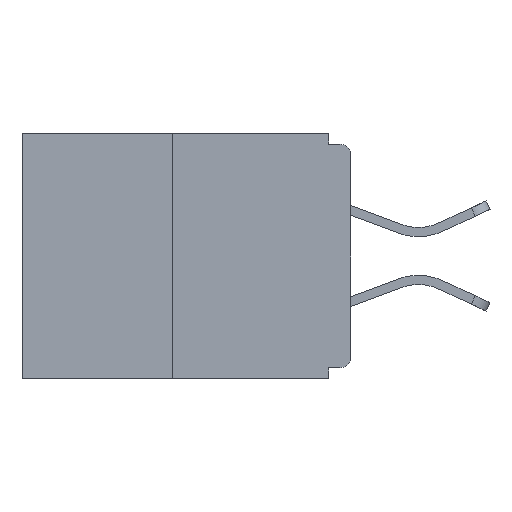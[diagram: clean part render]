
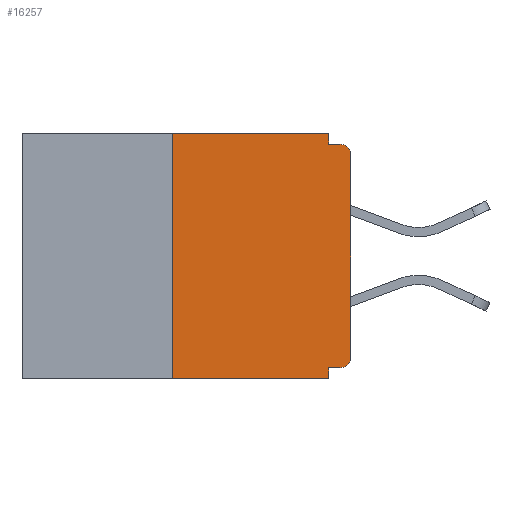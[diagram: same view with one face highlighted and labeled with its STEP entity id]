
A CAD part, left-side view. The second image highlights one B-rep face of the part: STEP entity #16257.
In plain terms, the highlighted planar face has unit normal (-1, 0, 0).
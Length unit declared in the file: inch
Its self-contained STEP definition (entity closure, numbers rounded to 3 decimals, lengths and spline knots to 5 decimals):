
#686 = CARTESIAN_POINT ( 'NONE',  ( 0., 0.015, -0.03 ) ) ;
#1086 = LINE ( 'NONE', #7236, #3591 ) ;
#1293 = LINE ( 'NONE', #18063, #6574 ) ;
#1392 = VERTEX_POINT ( 'NONE', #3799 ) ;
#1518 = VERTEX_POINT ( 'NONE', #22064 ) ;
#2824 = DIRECTION ( 'NONE',  ( 0., -1., 0. ) ) ;
#2896 = CARTESIAN_POINT ( 'NONE',  ( 0., 0.25, 0. ) ) ;
#3111 = EDGE_LOOP ( 'NONE', ( #5064, #6084, #10311, #18192, #11988, #22037, #6986, #12767, #12832, #10343 ) ) ;
#3137 = CARTESIAN_POINT ( 'NONE',  ( 0., 0.46, 0. ) ) ;
#3256 = DIRECTION ( 'NONE',  ( 0., -1., 0. ) ) ;
#3439 = VECTOR ( 'NONE', #3256, 39.37008 ) ;
#3578 = VERTEX_POINT ( 'NONE', #11507 ) ;
#3591 = VECTOR ( 'NONE', #17763, 39.37008 ) ;
#3665 = CIRCLE ( 'NONE', #6596, 0.015 ) ;
#3799 = CARTESIAN_POINT ( 'NONE',  ( 0., 0.015, -0.015 ) ) ;
#3884 = VERTEX_POINT ( 'NONE', #17634 ) ;
#4824 = LINE ( 'NONE', #15716, #3439 ) ;
#5027 = CIRCLE ( 'NONE', #20425, 0.015 ) ;
#5064 = ORIENTED_EDGE ( 'NONE', *, *, #16076, .F. ) ;
#5267 = CARTESIAN_POINT ( 'NONE',  ( 0., 0., -0.015 ) ) ;
#6084 = ORIENTED_EDGE ( 'NONE', *, *, #14226, .F. ) ;
#6134 = VERTEX_POINT ( 'NONE', #9829 ) ;
#6143 = VERTEX_POINT ( 'NONE', #20132 ) ;
#6296 = VERTEX_POINT ( 'NONE', #13304 ) ;
#6304 = LINE ( 'NONE', #5267, #15314 ) ;
#6574 = VECTOR ( 'NONE', #15235, 39.37008 ) ;
#6596 = AXIS2_PLACEMENT_3D ( 'NONE', #21957, #20246, #11429 ) ;
#6986 = ORIENTED_EDGE ( 'NONE', *, *, #22773, .T. ) ;
#7236 = CARTESIAN_POINT ( 'NONE',  ( 0., 0., 0. ) ) ;
#7850 = DIRECTION ( 'NONE',  ( 0., 0., -1. ) ) ;
#8027 = DIRECTION ( 'NONE',  ( -1., 0., 0. ) ) ;
#8207 = DIRECTION ( 'NONE',  ( 0., 0., -1. ) ) ;
#9172 = DIRECTION ( 'NONE',  ( 0., 0., 1. ) ) ;
#9654 = LINE ( 'NONE', #3137, #20111 ) ;
#9720 = EDGE_CURVE ( 'NONE', #6143, #1392, #6304, .T. ) ;
#9829 = CARTESIAN_POINT ( 'NONE',  ( 0., 0.015, -0.328 ) ) ;
#10311 = ORIENTED_EDGE ( 'NONE', *, *, #19846, .T. ) ;
#10343 = ORIENTED_EDGE ( 'NONE', *, *, #17300, .F. ) ;
#11187 = VERTEX_POINT ( 'NONE', #13243 ) ;
#11429 = DIRECTION ( 'NONE',  ( 0., 0., -1. ) ) ;
#11507 = CARTESIAN_POINT ( 'NONE',  ( 0., 0.031, 0. ) ) ;
#11532 = PLANE ( 'NONE',  #16523 ) ;
#11988 = ORIENTED_EDGE ( 'NONE', *, *, #12047, .F. ) ;
#12047 = EDGE_CURVE ( 'NONE', #6134, #3884, #17233, .T. ) ;
#12199 = DIRECTION ( 'NONE',  ( 0., 1., 0. ) ) ;
#12627 = CARTESIAN_POINT ( 'NONE',  ( 0., 0.031, -0.343 ) ) ;
#12767 = ORIENTED_EDGE ( 'NONE', *, *, #21464, .T. ) ;
#12832 = ORIENTED_EDGE ( 'NONE', *, *, #9720, .F. ) ;
#13243 = CARTESIAN_POINT ( 'NONE',  ( 0., 0.25, -0.343 ) ) ;
#13304 = CARTESIAN_POINT ( 'NONE',  ( 0., 0., -0.03 ) ) ;
#13454 = FACE_OUTER_BOUND ( 'NONE', #3111, .T. ) ;
#13843 = VERTEX_POINT ( 'NONE', #12627 ) ;
#14226 = EDGE_CURVE ( 'NONE', #11187, #16064, #19319, .T. ) ;
#15235 = DIRECTION ( 'NONE',  ( 0., 0., -1. ) ) ;
#15314 = VECTOR ( 'NONE', #15618, 39.37008 ) ;
#15618 = DIRECTION ( 'NONE',  ( 0., -1., 0. ) ) ;
#15716 = CARTESIAN_POINT ( 'NONE',  ( 0., 0.46, -0.343 ) ) ;
#16064 = VERTEX_POINT ( 'NONE', #2896 ) ;
#16076 = EDGE_CURVE ( 'NONE', #16064, #3578, #9654, .T. ) ;
#16257 = ADVANCED_FACE ( 'NONE', ( #13454 ), #11532, .F. ) ;
#16523 = AXIS2_PLACEMENT_3D ( 'NONE', #20359, #16613, #7850 ) ;
#16613 = DIRECTION ( 'NONE',  ( 1., 0., 0. ) ) ;
#16784 = DIRECTION ( 'NONE',  ( 0., 0., -1. ) ) ;
#16900 = CARTESIAN_POINT ( 'NONE',  ( 0., 0.031, -0.343 ) ) ;
#17233 = LINE ( 'NONE', #22741, #20232 ) ;
#17300 = EDGE_CURVE ( 'NONE', #3578, #6143, #1293, .T. ) ;
#17500 = VECTOR ( 'NONE', #8207, 39.37008 ) ;
#17634 = CARTESIAN_POINT ( 'NONE',  ( 0., 0.031, -0.328 ) ) ;
#17763 = DIRECTION ( 'NONE',  ( 0., 0., 1. ) ) ;
#18063 = CARTESIAN_POINT ( 'NONE',  ( 0., 0.031, 0. ) ) ;
#18192 = ORIENTED_EDGE ( 'NONE', *, *, #19830, .F. ) ;
#19319 = LINE ( 'NONE', #19696, #20688 ) ;
#19696 = CARTESIAN_POINT ( 'NONE',  ( 0., 0.25, 0. ) ) ;
#19830 = EDGE_CURVE ( 'NONE', #3884, #13843, #21344, .T. ) ;
#19846 = EDGE_CURVE ( 'NONE', #11187, #13843, #4824, .T. ) ;
#20111 = VECTOR ( 'NONE', #2824, 39.37008 ) ;
#20132 = CARTESIAN_POINT ( 'NONE',  ( 0., 0.031, -0.015 ) ) ;
#20232 = VECTOR ( 'NONE', #12199, 39.37008 ) ;
#20246 = DIRECTION ( 'NONE',  ( -1., 0., 0. ) ) ;
#20359 = CARTESIAN_POINT ( 'NONE',  ( 0., 0.46, 0. ) ) ;
#20425 = AXIS2_PLACEMENT_3D ( 'NONE', #686, #8027, #16784 ) ;
#20688 = VECTOR ( 'NONE', #9172, 39.37008 ) ;
#21344 = LINE ( 'NONE', #16900, #17500 ) ;
#21446 = EDGE_CURVE ( 'NONE', #6134, #1518, #3665, .T. ) ;
#21464 = EDGE_CURVE ( 'NONE', #6296, #1392, #5027, .T. ) ;
#21957 = CARTESIAN_POINT ( 'NONE',  ( 0., 0.015, -0.313 ) ) ;
#22037 = ORIENTED_EDGE ( 'NONE', *, *, #21446, .T. ) ;
#22064 = CARTESIAN_POINT ( 'NONE',  ( 0., 0., -0.313 ) ) ;
#22741 = CARTESIAN_POINT ( 'NONE',  ( 0., 0., -0.328 ) ) ;
#22773 = EDGE_CURVE ( 'NONE', #1518, #6296, #1086, .T. ) ;
